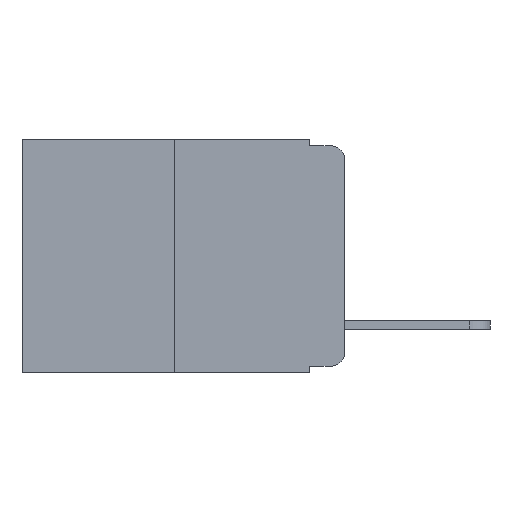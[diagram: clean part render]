
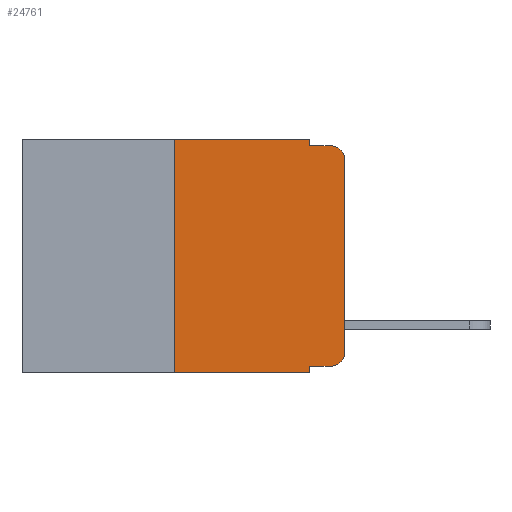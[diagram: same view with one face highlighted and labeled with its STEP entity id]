
A CAD part, left-side view. The second image highlights one B-rep face of the part: STEP entity #24761.
In plain terms, the highlighted planar face has unit normal (-1, 0, 0).
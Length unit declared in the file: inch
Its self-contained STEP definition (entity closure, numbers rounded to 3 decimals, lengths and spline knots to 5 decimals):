
#154 = CARTESIAN_POINT ( 'NONE',  ( 0., 0.473, 0. ) ) ;
#210 = VERTEX_POINT ( 'NONE', #11075 ) ;
#315 = VERTEX_POINT ( 'NONE', #2204 ) ;
#1589 = VERTEX_POINT ( 'NONE', #20982 ) ;
#2204 = CARTESIAN_POINT ( 'NONE',  ( 0., 0., -0.03 ) ) ;
#2435 = CIRCLE ( 'NONE', #21547, 0.02 ) ;
#2532 = DIRECTION ( 'NONE',  ( 0., 0., -1. ) ) ;
#3095 = VERTEX_POINT ( 'NONE', #24172 ) ;
#3122 = VECTOR ( 'NONE', #12872, 39.37008 ) ;
#3447 = EDGE_LOOP ( 'NONE', ( #11709, #12341, #12837, #12888, #13390, #14192, #14217, #16009, #16659, #16682 ) ) ;
#3469 = VECTOR ( 'NONE', #7453, 39.37008 ) ;
#4790 = CARTESIAN_POINT ( 'NONE',  ( 0., 0.051, 0. ) ) ;
#5156 = FACE_OUTER_BOUND ( 'NONE', #3447, .T. ) ;
#5211 = EDGE_CURVE ( 'NONE', #3095, #20720, #17895, .T. ) ;
#5356 = DIRECTION ( 'NONE',  ( 0., 0., -1. ) ) ;
#5417 = DIRECTION ( 'NONE',  ( -1., 0., 0. ) ) ;
#5531 = CARTESIAN_POINT ( 'NONE',  ( 0., 0.02, -0.313 ) ) ;
#6359 = EDGE_CURVE ( 'NONE', #7968, #315, #14594, .T. ) ;
#6405 = EDGE_CURVE ( 'NONE', #315, #1589, #2435, .T. ) ;
#6407 = EDGE_CURVE ( 'NONE', #14057, #1589, #22194, .T. ) ;
#6412 = EDGE_CURVE ( 'NONE', #23656, #14057, #21676, .T. ) ;
#6453 = EDGE_CURVE ( 'NONE', #3095, #19804, #19896, .T. ) ;
#6478 = EDGE_CURVE ( 'NONE', #19559, #20720, #9059, .T. ) ;
#6486 = EDGE_CURVE ( 'NONE', #19559, #210, #23492, .T. ) ;
#6527 = EDGE_CURVE ( 'NONE', #210, #7968, #17563, .T. ) ;
#7240 = DIRECTION ( 'NONE',  ( 0., -1., 0. ) ) ;
#7303 = CARTESIAN_POINT ( 'NONE',  ( 0., 0.051, -0.333 ) ) ;
#7453 = DIRECTION ( 'NONE',  ( 0., 0., -1. ) ) ;
#7820 = CARTESIAN_POINT ( 'NONE',  ( 0., 0.051, 0. ) ) ;
#7968 = VERTEX_POINT ( 'NONE', #12670 ) ;
#8046 = DIRECTION ( 'NONE',  ( 0., 0., 1. ) ) ;
#8396 = CARTESIAN_POINT ( 'NONE',  ( 0., 0.25, 0. ) ) ;
#8637 = VECTOR ( 'NONE', #21733, 39.37008 ) ;
#9059 = LINE ( 'NONE', #7820, #3469 ) ;
#9432 = DIRECTION ( 'NONE',  ( 0., 0., -1. ) ) ;
#9460 = CARTESIAN_POINT ( 'NONE',  ( 0., 0.051, 0. ) ) ;
#10250 = DIRECTION ( 'NONE',  ( 0., -1., 0. ) ) ;
#10277 = CARTESIAN_POINT ( 'NONE',  ( 0., 0.051, -0.01 ) ) ;
#10387 = DIRECTION ( 'NONE',  ( 0., 0., -1. ) ) ;
#10453 = DIRECTION ( 'NONE',  ( -1., 0., 0. ) ) ;
#10479 = CARTESIAN_POINT ( 'NONE',  ( 0., 0.02, -0.03 ) ) ;
#10827 = PLANE ( 'NONE',  #12413 ) ;
#11075 = CARTESIAN_POINT ( 'NONE',  ( 0., 0.02, -0.333 ) ) ;
#11709 = ORIENTED_EDGE ( 'NONE', *, *, #6359, .T. ) ;
#12304 = CARTESIAN_POINT ( 'NONE',  ( 0., 0.25, 0. ) ) ;
#12309 = CARTESIAN_POINT ( 'NONE',  ( 0., 0., 0. ) ) ;
#12341 = ORIENTED_EDGE ( 'NONE', *, *, #6405, .T. ) ;
#12413 = AXIS2_PLACEMENT_3D ( 'NONE', #154, #14774, #2532 ) ;
#12670 = CARTESIAN_POINT ( 'NONE',  ( 0., 0., -0.313 ) ) ;
#12837 = ORIENTED_EDGE ( 'NONE', *, *, #6407, .F. ) ;
#12872 = DIRECTION ( 'NONE',  ( 0., 0., 1. ) ) ;
#12888 = ORIENTED_EDGE ( 'NONE', *, *, #6412, .F. ) ;
#13390 = ORIENTED_EDGE ( 'NONE', *, *, #18095, .F. ) ;
#13722 = VECTOR ( 'NONE', #7240, 39.37008 ) ;
#14057 = VERTEX_POINT ( 'NONE', #21635 ) ;
#14192 = ORIENTED_EDGE ( 'NONE', *, *, #6453, .F. ) ;
#14217 = ORIENTED_EDGE ( 'NONE', *, *, #5211, .T. ) ;
#14594 = LINE ( 'NONE', #12309, #3122 ) ;
#14774 = DIRECTION ( 'NONE',  ( 1., 0., 0. ) ) ;
#14889 = VECTOR ( 'NONE', #8046, 39.37008 ) ;
#15903 = CARTESIAN_POINT ( 'NONE',  ( 0., 0.473, -0.343 ) ) ;
#15907 = DIRECTION ( 'NONE',  ( 0., -1., 0. ) ) ;
#16009 = ORIENTED_EDGE ( 'NONE', *, *, #6478, .F. ) ;
#16659 = ORIENTED_EDGE ( 'NONE', *, *, #6486, .T. ) ;
#16682 = ORIENTED_EDGE ( 'NONE', *, *, #6527, .T. ) ;
#17274 = VECTOR ( 'NONE', #9432, 39.37008 ) ;
#17284 = VECTOR ( 'NONE', #15907, 39.37008 ) ;
#17563 = CIRCLE ( 'NONE', #19809, 0.02 ) ;
#17590 = CARTESIAN_POINT ( 'NONE',  ( 0., 0.051, -0.333 ) ) ;
#17895 = LINE ( 'NONE', #15903, #17284 ) ;
#18095 = EDGE_CURVE ( 'NONE', #19804, #23656, #23675, .T. ) ;
#19559 = VERTEX_POINT ( 'NONE', #17590 ) ;
#19804 = VERTEX_POINT ( 'NONE', #12304 ) ;
#19809 = AXIS2_PLACEMENT_3D ( 'NONE', #5531, #5417, #5356 ) ;
#19896 = LINE ( 'NONE', #8396, #14889 ) ;
#20720 = VERTEX_POINT ( 'NONE', #20979 ) ;
#20979 = CARTESIAN_POINT ( 'NONE',  ( 0., 0.051, -0.343 ) ) ;
#20982 = CARTESIAN_POINT ( 'NONE',  ( 0., 0.02, -0.01 ) ) ;
#21547 = AXIS2_PLACEMENT_3D ( 'NONE', #10479, #10453, #10387 ) ;
#21635 = CARTESIAN_POINT ( 'NONE',  ( 0., 0.051, -0.01 ) ) ;
#21676 = LINE ( 'NONE', #9460, #17274 ) ;
#21733 = DIRECTION ( 'NONE',  ( 0., -1., 0. ) ) ;
#22194 = LINE ( 'NONE', #10277, #23236 ) ;
#23236 = VECTOR ( 'NONE', #10250, 39.37008 ) ;
#23416 = CARTESIAN_POINT ( 'NONE',  ( 0., 0.473, 0. ) ) ;
#23492 = LINE ( 'NONE', #7303, #13722 ) ;
#23656 = VERTEX_POINT ( 'NONE', #4790 ) ;
#23675 = LINE ( 'NONE', #23416, #8637 ) ;
#24172 = CARTESIAN_POINT ( 'NONE',  ( 0., 0.25, -0.343 ) ) ;
#24761 = ADVANCED_FACE ( 'NONE', ( #5156 ), #10827, .F. ) ;
